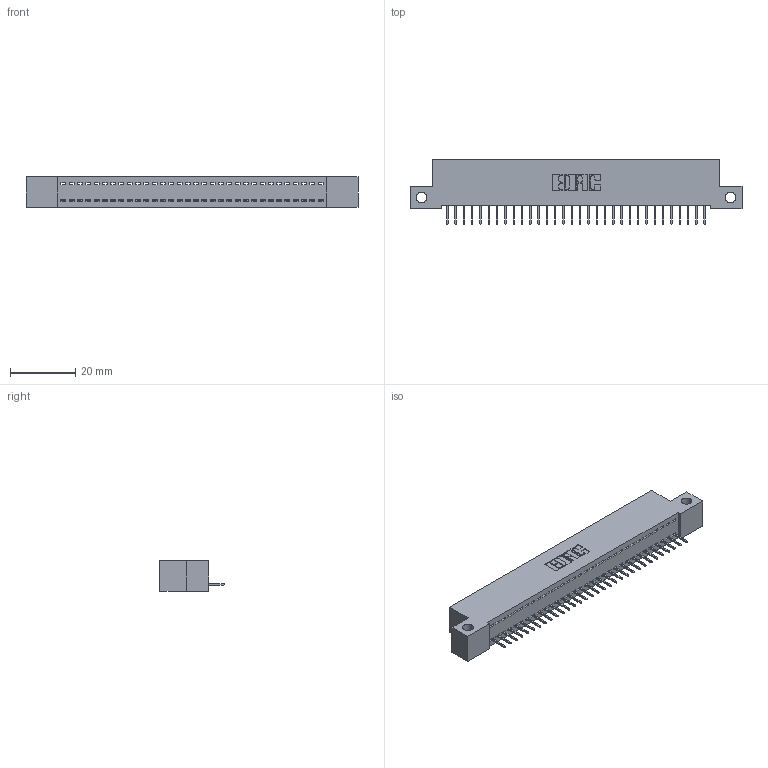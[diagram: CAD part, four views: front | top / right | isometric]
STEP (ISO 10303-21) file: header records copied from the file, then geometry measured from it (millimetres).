
FILE_DESCRIPTION (( 'STEP AP203' ), '1' );
FILE_NAME ('392-032-524-112.STEP', '2018-08-15T23:50:40', ( '' ), ( '' ), 'SwSTEP 2.0', 'SolidWorks 2016', '' );
FILE_SCHEMA (( 'CONFIG_CONTROL_DESIGN' ));
Length unit declared in the file: inch
Products named in the file (3): 342 Part_Side Mount; 345-292-001_345-293-124; 392-032-524-112
Assembly tree (33 placements, depth 2):
  392-032-524-112
    342 Part_Side Mount
    345-292-001_345-293-124  x32
Bounding box: 101.6 x 19.69 x 9.4 mm (x, y, z)
Volume: 8671.1 mm3; surface area: 11990.7 mm2
Topology: 33 solids, 33 shells, 2094 faces, 6059 edges, 3910 vertices
Faces by surface type: plane 1602, cylinder 492
Entity records: 20801 total; most frequent: CARTESIAN_POINT 3594, ORIENTED_EDGE 3562, DIRECTION 3053, EDGE_CURVE 1781, LINE 1657, VECTOR 1657, VERTEX_POINT 1182, AXIS2_PLACEMENT_3D 698
